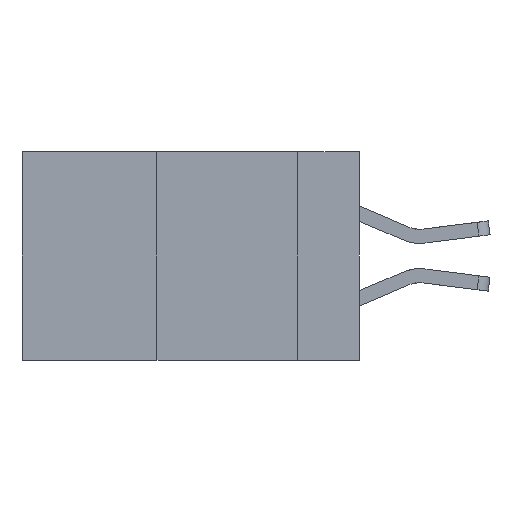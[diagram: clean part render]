
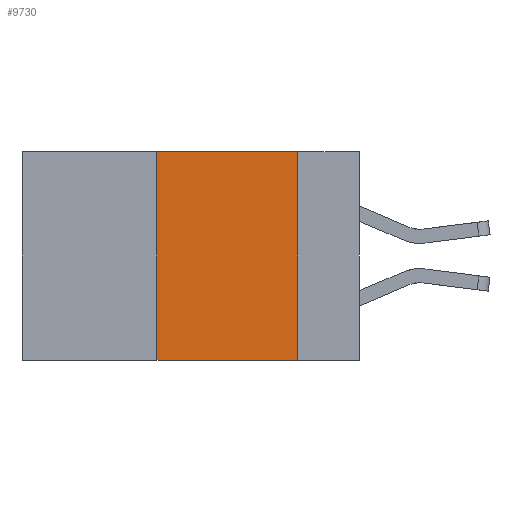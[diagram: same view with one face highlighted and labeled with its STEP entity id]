
A CAD part, left-side view. The second image highlights one B-rep face of the part: STEP entity #9730.
In plain terms, the highlighted planar face has unit normal (-1, 0, 0).
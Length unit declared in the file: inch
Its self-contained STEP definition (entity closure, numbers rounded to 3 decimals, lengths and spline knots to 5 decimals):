
#158 = CARTESIAN_POINT ( 'NONE',  ( 0., 0.6, -0.37 ) ) ;
#201 = VERTEX_POINT ( 'NONE', #8408 ) ;
#210 = VECTOR ( 'NONE', #3181, 39.37008 ) ;
#261 = EDGE_LOOP ( 'NONE', ( #2098, #1258, #7125, #6598 ) ) ;
#927 = DIRECTION ( 'NONE',  ( 0., 0., 1. ) ) ;
#975 = VERTEX_POINT ( 'NONE', #9351 ) ;
#1258 = ORIENTED_EDGE ( 'NONE', *, *, #1779, .F. ) ;
#1352 = CARTESIAN_POINT ( 'NONE',  ( 0., 0.11, -0.37 ) ) ;
#1537 = VECTOR ( 'NONE', #5909, 39.37008 ) ;
#1779 = EDGE_CURVE ( 'NONE', #201, #9348, #2903, .T. ) ;
#2093 = DIRECTION ( 'NONE',  ( 1., 0., 0. ) ) ;
#2098 = ORIENTED_EDGE ( 'NONE', *, *, #8837, .F. ) ;
#2218 = CARTESIAN_POINT ( 'NONE',  ( 0., 0.6, 0. ) ) ;
#2616 = EDGE_CURVE ( 'NONE', #975, #3608, #4015, .T. ) ;
#2885 = EDGE_CURVE ( 'NONE', #975, #201, #6823, .T. ) ;
#2903 = LINE ( 'NONE', #2218, #6843 ) ;
#3181 = DIRECTION ( 'NONE',  ( 0., -1., 0. ) ) ;
#3481 = FACE_OUTER_BOUND ( 'NONE', #261, .T. ) ;
#3608 = VERTEX_POINT ( 'NONE', #1352 ) ;
#4015 = LINE ( 'NONE', #158, #210 ) ;
#4918 = DIRECTION ( 'NONE',  ( 0., 0., -1. ) ) ;
#5028 = CARTESIAN_POINT ( 'NONE',  ( 0., 0.11, 0. ) ) ;
#5820 = CARTESIAN_POINT ( 'NONE',  ( 0., 0.11, 0. ) ) ;
#5909 = DIRECTION ( 'NONE',  ( 0., 0., -1. ) ) ;
#6020 = CARTESIAN_POINT ( 'NONE',  ( 0., 0.36, 0. ) ) ;
#6054 = VECTOR ( 'NONE', #927, 39.37008 ) ;
#6469 = LINE ( 'NONE', #5820, #1537 ) ;
#6598 = ORIENTED_EDGE ( 'NONE', *, *, #2616, .T. ) ;
#6823 = LINE ( 'NONE', #6020, #6054 ) ;
#6843 = VECTOR ( 'NONE', #9684, 39.37008 ) ;
#7125 = ORIENTED_EDGE ( 'NONE', *, *, #2885, .F. ) ;
#7286 = PLANE ( 'NONE',  #7397 ) ;
#7397 = AXIS2_PLACEMENT_3D ( 'NONE', #8835, #2093, #4918 ) ;
#8408 = CARTESIAN_POINT ( 'NONE',  ( 0., 0.36, 0. ) ) ;
#8835 = CARTESIAN_POINT ( 'NONE',  ( 0., 0.6, 0. ) ) ;
#8837 = EDGE_CURVE ( 'NONE', #9348, #3608, #6469, .T. ) ;
#9348 = VERTEX_POINT ( 'NONE', #5028 ) ;
#9351 = CARTESIAN_POINT ( 'NONE',  ( 0., 0.36, -0.37 ) ) ;
#9684 = DIRECTION ( 'NONE',  ( 0., -1., 0. ) ) ;
#9730 = ADVANCED_FACE ( 'NONE', ( #3481 ), #7286, .F. ) ;
